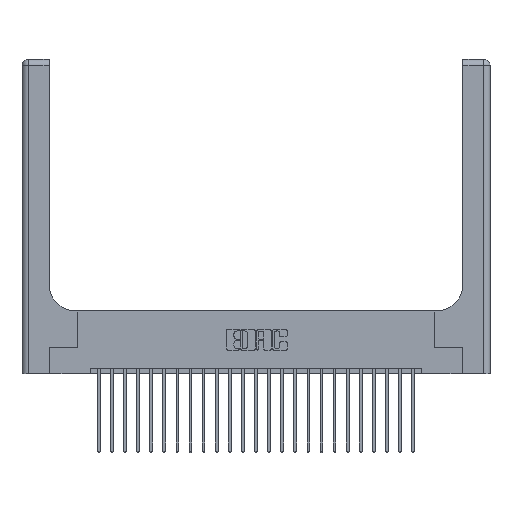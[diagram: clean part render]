
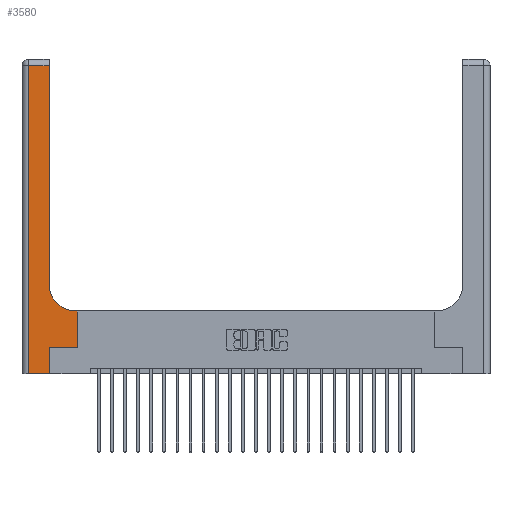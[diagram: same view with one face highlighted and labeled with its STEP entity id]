
A CAD part, top view. The second image highlights one B-rep face of the part: STEP entity #3580.
In plain terms, the highlighted planar face has unit normal (0, 0, 1).
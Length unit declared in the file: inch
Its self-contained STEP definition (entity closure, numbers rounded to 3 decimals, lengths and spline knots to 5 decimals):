
#409 = EDGE_CURVE ( 'NONE', #17360, #2120, #1494, .T. ) ;
#454 = EDGE_LOOP ( 'NONE', ( #10638, #17224, #1679, #5841, #22616, #19650, #15398, #21656, #5355 ) ) ;
#582 = LINE ( 'NONE', #14980, #917 ) ;
#803 = CARTESIAN_POINT ( 'NONE',  ( 0.26, 0.85, 0.37 ) ) ;
#917 = VECTOR ( 'NONE', #5626, 39.37008 ) ;
#1393 = DIRECTION ( 'NONE',  ( -1., 0., 0. ) ) ;
#1494 = LINE ( 'NONE', #16722, #1628 ) ;
#1628 = VECTOR ( 'NONE', #18802, 39.37008 ) ;
#1679 = ORIENTED_EDGE ( 'NONE', *, *, #5135, .T. ) ;
#1836 = CARTESIAN_POINT ( 'NONE',  ( 0.06, 3., 0.37 ) ) ;
#2079 = VECTOR ( 'NONE', #19165, 39.37008 ) ;
#2120 = VERTEX_POINT ( 'NONE', #18778 ) ;
#2327 = VECTOR ( 'NONE', #1393, 39.37008 ) ;
#2360 = VERTEX_POINT ( 'NONE', #23064 ) ;
#2509 = CIRCLE ( 'NONE', #6827, 0.25 ) ;
#3036 = EDGE_CURVE ( 'NONE', #3327, #21809, #22023, .T. ) ;
#3327 = VERTEX_POINT ( 'NONE', #14302 ) ;
#3580 = ADVANCED_FACE ( 'NONE', ( #6639 ), #17804, .F. ) ;
#4574 = DIRECTION ( 'NONE',  ( 0., 1., 0. ) ) ;
#5038 = VERTEX_POINT ( 'NONE', #20017 ) ;
#5135 = EDGE_CURVE ( 'NONE', #5038, #2360, #20835, .T. ) ;
#5355 = ORIENTED_EDGE ( 'NONE', *, *, #8309, .T. ) ;
#5626 = DIRECTION ( 'NONE',  ( 0., 1., 0. ) ) ;
#5841 = ORIENTED_EDGE ( 'NONE', *, *, #18575, .T. ) ;
#6267 = CARTESIAN_POINT ( 'NONE',  ( 0.265, 0., 0.37 ) ) ;
#6639 = FACE_OUTER_BOUND ( 'NONE', #454, .T. ) ;
#6827 = AXIS2_PLACEMENT_3D ( 'NONE', #13771, #17674, #17917 ) ;
#8247 = DIRECTION ( 'NONE',  ( 0., 0., -1. ) ) ;
#8309 = EDGE_CURVE ( 'NONE', #21809, #22453, #2509, .T. ) ;
#8793 = CARTESIAN_POINT ( 'NONE',  ( 0., 0., 0.37 ) ) ;
#10638 = ORIENTED_EDGE ( 'NONE', *, *, #14818, .T. ) ;
#11760 = CARTESIAN_POINT ( 'NONE',  ( 0.26, 2.94, 0.37 ) ) ;
#12617 = DIRECTION ( 'NONE',  ( -1., 0., 0. ) ) ;
#12696 = CARTESIAN_POINT ( 'NONE',  ( 0.265, 0.25, 0.37 ) ) ;
#13771 = CARTESIAN_POINT ( 'NONE',  ( 0.51, 0.85, 0.37 ) ) ;
#13955 = AXIS2_PLACEMENT_3D ( 'NONE', #17689, #8247, #17438 ) ;
#14302 = CARTESIAN_POINT ( 'NONE',  ( 0.528, 0.6, 0.37 ) ) ;
#14818 = EDGE_CURVE ( 'NONE', #22453, #19538, #15756, .T. ) ;
#14980 = CARTESIAN_POINT ( 'NONE',  ( 0.528, 0.25, 0.37 ) ) ;
#15105 = CARTESIAN_POINT ( 'NONE',  ( 0.51, 0.6, 0.37 ) ) ;
#15398 = ORIENTED_EDGE ( 'NONE', *, *, #18003, .T. ) ;
#15403 = VERTEX_POINT ( 'NONE', #18849 ) ;
#15756 = LINE ( 'NONE', #19423, #15947 ) ;
#15903 = EDGE_CURVE ( 'NONE', #19538, #5038, #18344, .T. ) ;
#15947 = VECTOR ( 'NONE', #4574, 39.37008 ) ;
#16345 = VECTOR ( 'NONE', #22695, 39.37008 ) ;
#16722 = CARTESIAN_POINT ( 'NONE',  ( 0.265, 0.25, 0.37 ) ) ;
#17224 = ORIENTED_EDGE ( 'NONE', *, *, #15903, .T. ) ;
#17360 = VERTEX_POINT ( 'NONE', #12696 ) ;
#17438 = DIRECTION ( 'NONE',  ( -1., 0., 0. ) ) ;
#17674 = DIRECTION ( 'NONE',  ( 0., 0., -1. ) ) ;
#17689 = CARTESIAN_POINT ( 'NONE',  ( 0., 3., 0.37 ) ) ;
#17804 = PLANE ( 'NONE',  #13955 ) ;
#17917 = DIRECTION ( 'NONE',  ( 1., 0., 0. ) ) ;
#18003 = EDGE_CURVE ( 'NONE', #2120, #3327, #582, .T. ) ;
#18230 = DIRECTION ( 'NONE',  ( 1., 0., 0. ) ) ;
#18344 = LINE ( 'NONE', #24092, #2327 ) ;
#18575 = EDGE_CURVE ( 'NONE', #2360, #15403, #21918, .T. ) ;
#18778 = CARTESIAN_POINT ( 'NONE',  ( 0.528, 0.25, 0.37 ) ) ;
#18802 = DIRECTION ( 'NONE',  ( 1., 0., 0. ) ) ;
#18849 = CARTESIAN_POINT ( 'NONE',  ( 0.265, 0., 0.37 ) ) ;
#19165 = DIRECTION ( 'NONE',  ( 0., 1., 0. ) ) ;
#19423 = CARTESIAN_POINT ( 'NONE',  ( 0.26, 3., 0.37 ) ) ;
#19538 = VERTEX_POINT ( 'NONE', #11760 ) ;
#19650 = ORIENTED_EDGE ( 'NONE', *, *, #409, .T. ) ;
#19771 = VECTOR ( 'NONE', #12617, 39.37008 ) ;
#20017 = CARTESIAN_POINT ( 'NONE',  ( 0.06, 2.94, 0.37 ) ) ;
#20169 = EDGE_CURVE ( 'NONE', #15403, #17360, #23200, .T. ) ;
#20835 = LINE ( 'NONE', #1836, #16345 ) ;
#20998 = VECTOR ( 'NONE', #18230, 39.37008 ) ;
#21656 = ORIENTED_EDGE ( 'NONE', *, *, #3036, .T. ) ;
#21809 = VERTEX_POINT ( 'NONE', #15105 ) ;
#21918 = LINE ( 'NONE', #8793, #20998 ) ;
#22023 = LINE ( 'NONE', #23753, #19771 ) ;
#22453 = VERTEX_POINT ( 'NONE', #803 ) ;
#22616 = ORIENTED_EDGE ( 'NONE', *, *, #20169, .T. ) ;
#22695 = DIRECTION ( 'NONE',  ( 0., -1., 0. ) ) ;
#23064 = CARTESIAN_POINT ( 'NONE',  ( 0.06, 0., 0.37 ) ) ;
#23200 = LINE ( 'NONE', #6267, #2079 ) ;
#23753 = CARTESIAN_POINT ( 'NONE',  ( 0.26, 0.6, 0.37 ) ) ;
#24092 = CARTESIAN_POINT ( 'NONE',  ( 0., 2.94, 0.37 ) ) ;
